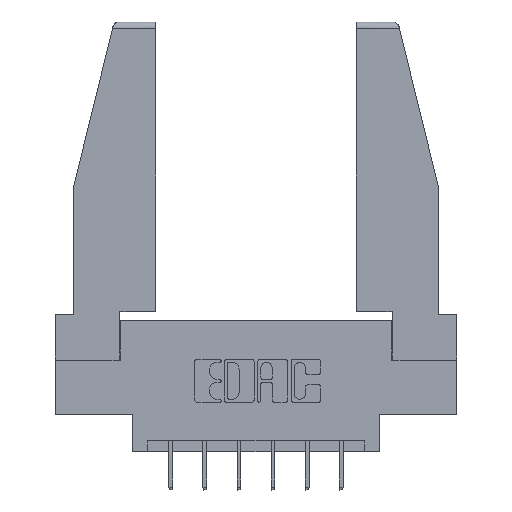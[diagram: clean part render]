
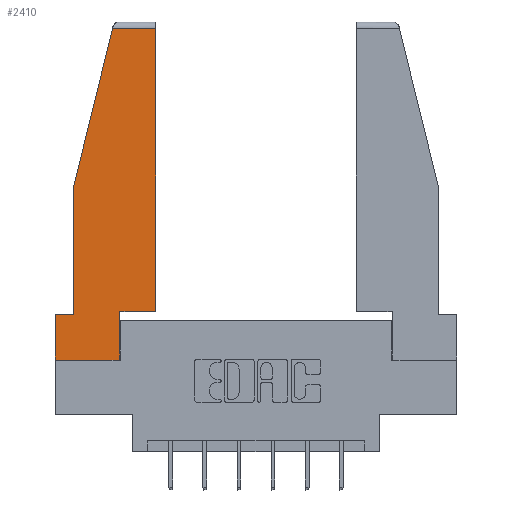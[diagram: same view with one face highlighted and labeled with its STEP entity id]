
A CAD part, top view. The second image highlights one B-rep face of the part: STEP entity #2410.
In plain terms, the highlighted planar face has unit normal (0, 0, 1).
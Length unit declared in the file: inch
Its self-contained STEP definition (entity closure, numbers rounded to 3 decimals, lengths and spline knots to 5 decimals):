
#72 = ORIENTED_EDGE ( 'NONE', *, *, #8777, .T. ) ;
#229 = VERTEX_POINT ( 'NONE', #5578 ) ;
#321 = ORIENTED_EDGE ( 'NONE', *, *, #9926, .T. ) ;
#510 = EDGE_LOOP ( 'NONE', ( #72, #4760, #10088, #11103, #9053, #7616, #592, #5985, #321 ) ) ;
#592 = ORIENTED_EDGE ( 'NONE', *, *, #1130, .T. ) ;
#799 = EDGE_CURVE ( 'NONE', #10024, #5426, #7057, .T. ) ;
#826 = PLANE ( 'NONE',  #6413 ) ;
#1130 = EDGE_CURVE ( 'NONE', #4699, #9491, #11569, .T. ) ;
#1682 = LINE ( 'NONE', #11116, #11541 ) ;
#1696 = EDGE_CURVE ( 'NONE', #9989, #10024, #6918, .T. ) ;
#1777 = LINE ( 'NONE', #4923, #10504 ) ;
#2372 = VERTEX_POINT ( 'NONE', #5680 ) ;
#2410 = ADVANCED_FACE ( 'NONE', ( #3272 ), #826, .T. ) ;
#2693 = CARTESIAN_POINT ( 'NONE',  ( 0.086, 0.21, 0. ) ) ;
#2754 = DIRECTION ( 'NONE',  ( 1., 0., 0. ) ) ;
#2987 = DIRECTION ( 'NONE',  ( -0.239, -0.971, 0. ) ) ;
#3272 = FACE_OUTER_BOUND ( 'NONE', #510, .T. ) ;
#3542 = CARTESIAN_POINT ( 'NONE',  ( 0.086, 0.8, 0. ) ) ;
#3985 = VECTOR ( 'NONE', #5287, 39.37008 ) ;
#4227 = VECTOR ( 'NONE', #11588, 39.37008 ) ;
#4260 = CARTESIAN_POINT ( 'NONE',  ( 0.297, 0.223, 0. ) ) ;
#4585 = CARTESIAN_POINT ( 'NONE',  ( 0.297, 0., 0. ) ) ;
#4588 = DIRECTION ( 'NONE',  ( 0., -1., 0. ) ) ;
#4698 = DIRECTION ( 'NONE',  ( 1., 0., 0. ) ) ;
#4699 = VERTEX_POINT ( 'NONE', #4767 ) ;
#4702 = DIRECTION ( 'NONE',  ( 0., 1., 0. ) ) ;
#4760 = ORIENTED_EDGE ( 'NONE', *, *, #4956, .T. ) ;
#4767 = CARTESIAN_POINT ( 'NONE',  ( 0., 0., 0. ) ) ;
#4923 = CARTESIAN_POINT ( 'NONE',  ( 0., 0.21, 0. ) ) ;
#4956 = EDGE_CURVE ( 'NONE', #11262, #9989, #11639, .T. ) ;
#5287 = DIRECTION ( 'NONE',  ( -1., 0., 0. ) ) ;
#5300 = EDGE_CURVE ( 'NONE', #9491, #7668, #8909, .T. ) ;
#5308 = EDGE_CURVE ( 'NONE', #2372, #4699, #1777, .T. ) ;
#5426 = VERTEX_POINT ( 'NONE', #2693 ) ;
#5578 = CARTESIAN_POINT ( 'NONE',  ( 0.461, 0.223, 0. ) ) ;
#5680 = CARTESIAN_POINT ( 'NONE',  ( 0., 0.21, 0. ) ) ;
#5985 = ORIENTED_EDGE ( 'NONE', *, *, #5300, .T. ) ;
#6350 = VECTOR ( 'NONE', #4702, 39.37008 ) ;
#6398 = VECTOR ( 'NONE', #11139, 39.37008 ) ;
#6413 = AXIS2_PLACEMENT_3D ( 'NONE', #7304, #9196, #2754 ) ;
#6508 = CARTESIAN_POINT ( 'NONE',  ( 0.297, 0., 0. ) ) ;
#6918 = LINE ( 'NONE', #8581, #10711 ) ;
#7057 = LINE ( 'NONE', #3542, #7222 ) ;
#7222 = VECTOR ( 'NONE', #4588, 39.37008 ) ;
#7304 = CARTESIAN_POINT ( 'NONE',  ( 0., 0., 0. ) ) ;
#7359 = CARTESIAN_POINT ( 'NONE',  ( 0.461, 0.223, 0. ) ) ;
#7616 = ORIENTED_EDGE ( 'NONE', *, *, #5308, .T. ) ;
#7647 = CARTESIAN_POINT ( 'NONE',  ( 0.086, 0.8, 0. ) ) ;
#7668 = VERTEX_POINT ( 'NONE', #4260 ) ;
#8581 = CARTESIAN_POINT ( 'NONE',  ( 0.271, 1.55, 0. ) ) ;
#8686 = DIRECTION ( 'NONE',  ( 0., -1., 0. ) ) ;
#8708 = CARTESIAN_POINT ( 'NONE',  ( 0.461, 1.52, 0. ) ) ;
#8777 = EDGE_CURVE ( 'NONE', #229, #11262, #11287, .T. ) ;
#8909 = LINE ( 'NONE', #4585, #6398 ) ;
#9053 = ORIENTED_EDGE ( 'NONE', *, *, #10413, .T. ) ;
#9196 = DIRECTION ( 'NONE',  ( 0., 0., 1. ) ) ;
#9491 = VERTEX_POINT ( 'NONE', #6508 ) ;
#9569 = DIRECTION ( 'NONE',  ( 1., 0., 0. ) ) ;
#9926 = EDGE_CURVE ( 'NONE', #7668, #229, #1682, .T. ) ;
#9989 = VERTEX_POINT ( 'NONE', #11157 ) ;
#10024 = VERTEX_POINT ( 'NONE', #7647 ) ;
#10088 = ORIENTED_EDGE ( 'NONE', *, *, #1696, .T. ) ;
#10413 = EDGE_CURVE ( 'NONE', #5426, #2372, #11400, .T. ) ;
#10504 = VECTOR ( 'NONE', #8686, 39.37008 ) ;
#10687 = CARTESIAN_POINT ( 'NONE',  ( 0., 1.52, 0. ) ) ;
#10711 = VECTOR ( 'NONE', #2987, 39.37008 ) ;
#10854 = CARTESIAN_POINT ( 'NONE',  ( 0., 0.21, 0. ) ) ;
#11103 = ORIENTED_EDGE ( 'NONE', *, *, #799, .T. ) ;
#11116 = CARTESIAN_POINT ( 'NONE',  ( 0.297, 0.223, 0. ) ) ;
#11139 = DIRECTION ( 'NONE',  ( 0., 1., 0. ) ) ;
#11157 = CARTESIAN_POINT ( 'NONE',  ( 0.2636, 1.52, 0. ) ) ;
#11231 = CARTESIAN_POINT ( 'NONE',  ( 0., 0., 0. ) ) ;
#11262 = VERTEX_POINT ( 'NONE', #8708 ) ;
#11287 = LINE ( 'NONE', #7359, #6350 ) ;
#11400 = LINE ( 'NONE', #10854, #3985 ) ;
#11541 = VECTOR ( 'NONE', #4698, 39.37008 ) ;
#11569 = LINE ( 'NONE', #11231, #11707 ) ;
#11588 = DIRECTION ( 'NONE',  ( -1., 0., 0. ) ) ;
#11639 = LINE ( 'NONE', #10687, #4227 ) ;
#11707 = VECTOR ( 'NONE', #9569, 39.37008 ) ;
